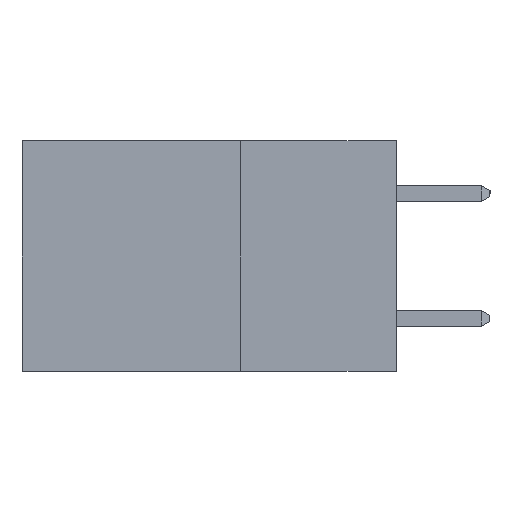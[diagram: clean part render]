
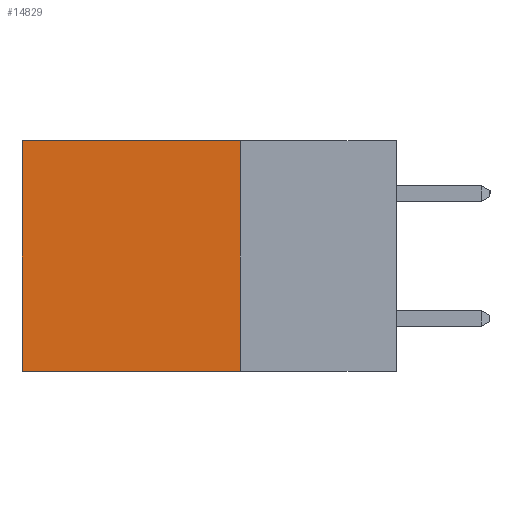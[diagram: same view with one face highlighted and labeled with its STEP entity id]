
A CAD part, left-side view. The second image highlights one B-rep face of the part: STEP entity #14829.
In plain terms, the highlighted planar face has unit normal (-1, 0, 0).
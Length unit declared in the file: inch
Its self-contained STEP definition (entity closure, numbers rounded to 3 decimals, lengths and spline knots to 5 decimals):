
#987 = LINE ( 'NONE', #18463, #18423 ) ;
#1639 = CARTESIAN_POINT ( 'NONE',  ( 0.2615, 0.25, -0.37 ) ) ;
#1881 = DIRECTION ( 'NONE',  ( 0., 0., -1. ) ) ;
#2214 = EDGE_LOOP ( 'NONE', ( #6633, #18999, #19144, #9377 ) ) ;
#2282 = VECTOR ( 'NONE', #4786, 39.37008 ) ;
#2920 = VERTEX_POINT ( 'NONE', #5766 ) ;
#3568 = LINE ( 'NONE', #10020, #6860 ) ;
#3762 = EDGE_CURVE ( 'NONE', #2920, #19755, #19314, .T. ) ;
#3843 = DIRECTION ( 'NONE',  ( 0., 0., -1. ) ) ;
#4786 = DIRECTION ( 'NONE',  ( 0., 1., 0. ) ) ;
#4925 = LINE ( 'NONE', #9899, #18248 ) ;
#5392 = VERTEX_POINT ( 'NONE', #17831 ) ;
#5573 = VERTEX_POINT ( 'NONE', #18866 ) ;
#5766 = CARTESIAN_POINT ( 'NONE',  ( 0.2615, 0.25, -0.37 ) ) ;
#6247 = EDGE_CURVE ( 'NONE', #5392, #5573, #4925, .T. ) ;
#6358 = CARTESIAN_POINT ( 'NONE',  ( 0.2615, 0.6, -0.37 ) ) ;
#6633 = ORIENTED_EDGE ( 'NONE', *, *, #10433, .T. ) ;
#6860 = VECTOR ( 'NONE', #1881, 39.37008 ) ;
#9377 = ORIENTED_EDGE ( 'NONE', *, *, #6247, .T. ) ;
#9899 = CARTESIAN_POINT ( 'NONE',  ( 0.2615, 0.25, 0. ) ) ;
#10020 = CARTESIAN_POINT ( 'NONE',  ( 0.2615, 0.6, -0.37 ) ) ;
#10433 = EDGE_CURVE ( 'NONE', #5573, #19755, #3568, .T. ) ;
#12880 = CARTESIAN_POINT ( 'NONE',  ( 0.2615, 0.25, -0.37 ) ) ;
#14346 = FACE_OUTER_BOUND ( 'NONE', #2214, .T. ) ;
#14829 = ADVANCED_FACE ( 'NONE', ( #14346 ), #20596, .F. ) ;
#16760 = AXIS2_PLACEMENT_3D ( 'NONE', #12880, #20697, #19014 ) ;
#17831 = CARTESIAN_POINT ( 'NONE',  ( 0.2615, 0.25, 0. ) ) ;
#18248 = VECTOR ( 'NONE', #19655, 39.37008 ) ;
#18423 = VECTOR ( 'NONE', #3843, 39.37008 ) ;
#18463 = CARTESIAN_POINT ( 'NONE',  ( 0.2615, 0.25, -0.37 ) ) ;
#18866 = CARTESIAN_POINT ( 'NONE',  ( 0.2615, 0.6, 0. ) ) ;
#18906 = EDGE_CURVE ( 'NONE', #5392, #2920, #987, .T. ) ;
#18999 = ORIENTED_EDGE ( 'NONE', *, *, #3762, .F. ) ;
#19014 = DIRECTION ( 'NONE',  ( 0., 0., -1. ) ) ;
#19144 = ORIENTED_EDGE ( 'NONE', *, *, #18906, .F. ) ;
#19314 = LINE ( 'NONE', #1639, #2282 ) ;
#19655 = DIRECTION ( 'NONE',  ( 0., 1., 0. ) ) ;
#19755 = VERTEX_POINT ( 'NONE', #6358 ) ;
#20596 = PLANE ( 'NONE',  #16760 ) ;
#20697 = DIRECTION ( 'NONE',  ( 1., 0., 0. ) ) ;
